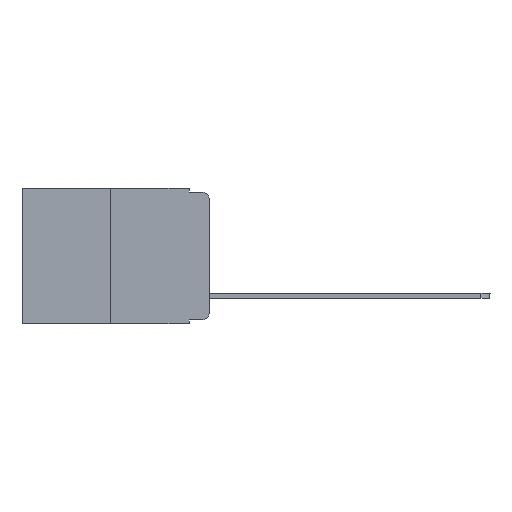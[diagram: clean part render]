
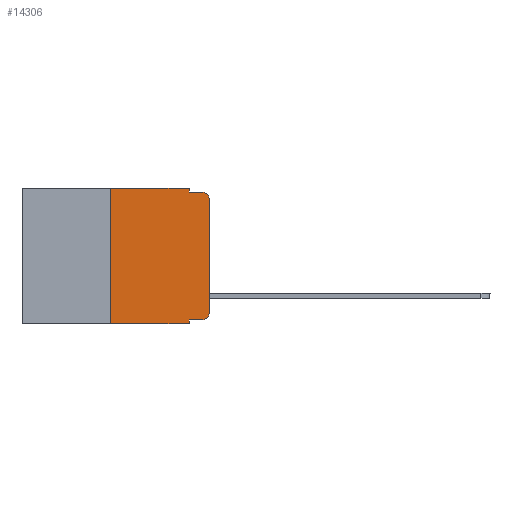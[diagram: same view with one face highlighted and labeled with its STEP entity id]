
A CAD part, left-side view. The second image highlights one B-rep face of the part: STEP entity #14306.
In plain terms, the highlighted planar face has unit normal (-1, 0, 0).
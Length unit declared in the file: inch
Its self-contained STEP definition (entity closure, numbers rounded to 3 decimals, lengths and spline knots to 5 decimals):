
#24 = VECTOR ( 'NONE', #796, 39.37008 ) ;
#417 = LINE ( 'NONE', #13609, #9389 ) ;
#432 = ORIENTED_EDGE ( 'NONE', *, *, #10525, .T. ) ;
#796 = DIRECTION ( 'NONE',  ( 0., 0., -1. ) ) ;
#823 = VERTEX_POINT ( 'NONE', #13279 ) ;
#1236 = ORIENTED_EDGE ( 'NONE', *, *, #5514, .T. ) ;
#1270 = VERTEX_POINT ( 'NONE', #12729 ) ;
#1288 = VECTOR ( 'NONE', #13011, 39.37008 ) ;
#1293 = CARTESIAN_POINT ( 'NONE',  ( 0., 0.051, -0.01 ) ) ;
#1769 = ORIENTED_EDGE ( 'NONE', *, *, #11598, .F. ) ;
#2069 = CARTESIAN_POINT ( 'NONE',  ( 0., 0.473, 0. ) ) ;
#2081 = CARTESIAN_POINT ( 'NONE',  ( 0., 0.473, 0. ) ) ;
#2277 = VERTEX_POINT ( 'NONE', #12391 ) ;
#2789 = VECTOR ( 'NONE', #2819, 39.37008 ) ;
#2819 = DIRECTION ( 'NONE',  ( 0., 0., -1. ) ) ;
#3361 = DIRECTION ( 'NONE',  ( 0., 0., -1. ) ) ;
#3439 = CARTESIAN_POINT ( 'NONE',  ( 0., 0.473, -0.343 ) ) ;
#3487 = VERTEX_POINT ( 'NONE', #4766 ) ;
#3528 = LINE ( 'NONE', #6211, #9407 ) ;
#3793 = DIRECTION ( 'NONE',  ( 0., 0., 1. ) ) ;
#3930 = CARTESIAN_POINT ( 'NONE',  ( 0., 0.02, -0.01 ) ) ;
#3963 = CARTESIAN_POINT ( 'NONE',  ( 0., 0.051, -0.01 ) ) ;
#4076 = LINE ( 'NONE', #9825, #2789 ) ;
#4090 = VECTOR ( 'NONE', #4530, 39.37008 ) ;
#4288 = DIRECTION ( 'NONE',  ( 0., 0., -1. ) ) ;
#4420 = CARTESIAN_POINT ( 'NONE',  ( 0., 0.051, -0.343 ) ) ;
#4427 = DIRECTION ( 'NONE',  ( 0., -1., 0. ) ) ;
#4442 = VERTEX_POINT ( 'NONE', #4420 ) ;
#4498 = ORIENTED_EDGE ( 'NONE', *, *, #5749, .T. ) ;
#4530 = DIRECTION ( 'NONE',  ( 0., -1., 0. ) ) ;
#4542 = PLANE ( 'NONE',  #5850 ) ;
#4766 = CARTESIAN_POINT ( 'NONE',  ( 0., 0., -0.313 ) ) ;
#4835 = EDGE_CURVE ( 'NONE', #13762, #9036, #8648, .T. ) ;
#4910 = CARTESIAN_POINT ( 'NONE',  ( 0., 0.25, 0. ) ) ;
#5009 = AXIS2_PLACEMENT_3D ( 'NONE', #6560, #11229, #4288 ) ;
#5416 = ORIENTED_EDGE ( 'NONE', *, *, #12398, .T. ) ;
#5473 = CIRCLE ( 'NONE', #6861, 0.02 ) ;
#5503 = CARTESIAN_POINT ( 'NONE',  ( 0., 0.02, -0.333 ) ) ;
#5514 = EDGE_CURVE ( 'NONE', #1270, #14126, #5473, .T. ) ;
#5726 = CARTESIAN_POINT ( 'NONE',  ( 0., 0.051, 0. ) ) ;
#5749 = EDGE_CURVE ( 'NONE', #823, #10710, #9745, .T. ) ;
#5850 = AXIS2_PLACEMENT_3D ( 'NONE', #2081, #10358, #3361 ) ;
#6143 = CARTESIAN_POINT ( 'NONE',  ( 0., 0.02, -0.03 ) ) ;
#6211 = CARTESIAN_POINT ( 'NONE',  ( 0., 0.25, 0. ) ) ;
#6560 = CARTESIAN_POINT ( 'NONE',  ( 0., 0.02, -0.313 ) ) ;
#6861 = AXIS2_PLACEMENT_3D ( 'NONE', #6143, #13318, #14373 ) ;
#7701 = ORIENTED_EDGE ( 'NONE', *, *, #9341, .T. ) ;
#7800 = CARTESIAN_POINT ( 'NONE',  ( 0., 0.051, 0. ) ) ;
#8151 = LINE ( 'NONE', #2069, #4090 ) ;
#8226 = LINE ( 'NONE', #3439, #12967 ) ;
#8456 = LINE ( 'NONE', #1293, #1288 ) ;
#8648 = LINE ( 'NONE', #7800, #24 ) ;
#9036 = VERTEX_POINT ( 'NONE', #3963 ) ;
#9178 = VECTOR ( 'NONE', #4427, 39.37008 ) ;
#9341 = EDGE_CURVE ( 'NONE', #2277, #4442, #8226, .T. ) ;
#9355 = DIRECTION ( 'NONE',  ( 0., -1., 0. ) ) ;
#9389 = VECTOR ( 'NONE', #13801, 39.37008 ) ;
#9407 = VECTOR ( 'NONE', #3793, 39.37008 ) ;
#9745 = LINE ( 'NONE', #11477, #9178 ) ;
#9814 = ORIENTED_EDGE ( 'NONE', *, *, #4835, .F. ) ;
#9825 = CARTESIAN_POINT ( 'NONE',  ( 0., 0.051, 0. ) ) ;
#10358 = DIRECTION ( 'NONE',  ( 1., 0., 0. ) ) ;
#10460 = FACE_OUTER_BOUND ( 'NONE', #13201, .T. ) ;
#10525 = EDGE_CURVE ( 'NONE', #10710, #3487, #13285, .T. ) ;
#10710 = VERTEX_POINT ( 'NONE', #5503 ) ;
#11051 = ORIENTED_EDGE ( 'NONE', *, *, #12636, .F. ) ;
#11211 = EDGE_CURVE ( 'NONE', #14032, #13762, #8151, .T. ) ;
#11229 = DIRECTION ( 'NONE',  ( -1., 0., 0. ) ) ;
#11477 = CARTESIAN_POINT ( 'NONE',  ( 0., 0.051, -0.333 ) ) ;
#11598 = EDGE_CURVE ( 'NONE', #823, #4442, #4076, .T. ) ;
#12391 = CARTESIAN_POINT ( 'NONE',  ( 0., 0.25, -0.343 ) ) ;
#12398 = EDGE_CURVE ( 'NONE', #3487, #1270, #417, .T. ) ;
#12636 = EDGE_CURVE ( 'NONE', #2277, #14032, #3528, .T. ) ;
#12729 = CARTESIAN_POINT ( 'NONE',  ( 0., 0., -0.03 ) ) ;
#12774 = ORIENTED_EDGE ( 'NONE', *, *, #13924, .F. ) ;
#12967 = VECTOR ( 'NONE', #9355, 39.37008 ) ;
#13011 = DIRECTION ( 'NONE',  ( 0., -1., 0. ) ) ;
#13201 = EDGE_LOOP ( 'NONE', ( #5416, #1236, #12774, #9814, #14183, #11051, #7701, #1769, #4498, #432 ) ) ;
#13279 = CARTESIAN_POINT ( 'NONE',  ( 0., 0.051, -0.333 ) ) ;
#13285 = CIRCLE ( 'NONE', #5009, 0.02 ) ;
#13318 = DIRECTION ( 'NONE',  ( -1., 0., 0. ) ) ;
#13609 = CARTESIAN_POINT ( 'NONE',  ( 0., 0., 0. ) ) ;
#13762 = VERTEX_POINT ( 'NONE', #5726 ) ;
#13801 = DIRECTION ( 'NONE',  ( 0., 0., 1. ) ) ;
#13924 = EDGE_CURVE ( 'NONE', #9036, #14126, #8456, .T. ) ;
#14032 = VERTEX_POINT ( 'NONE', #4910 ) ;
#14126 = VERTEX_POINT ( 'NONE', #3930 ) ;
#14183 = ORIENTED_EDGE ( 'NONE', *, *, #11211, .F. ) ;
#14306 = ADVANCED_FACE ( 'NONE', ( #10460 ), #4542, .F. ) ;
#14373 = DIRECTION ( 'NONE',  ( 0., 0., -1. ) ) ;
